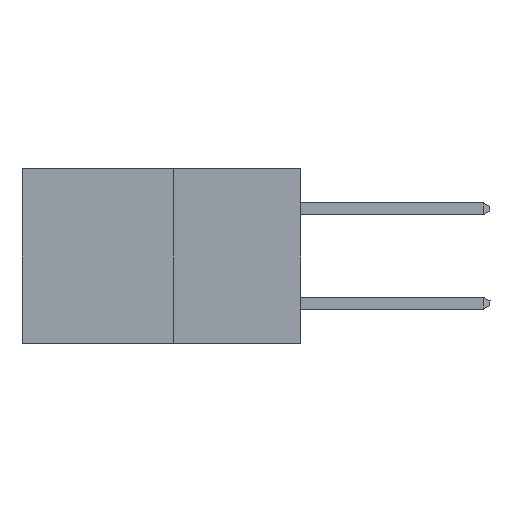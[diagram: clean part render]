
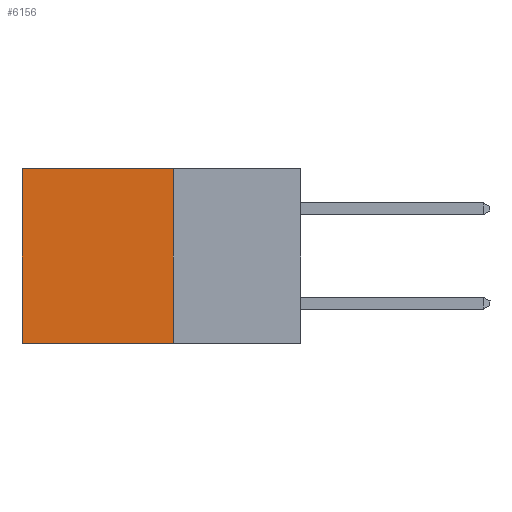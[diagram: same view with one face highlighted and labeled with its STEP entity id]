
A CAD part, left-side view. The second image highlights one B-rep face of the part: STEP entity #6156.
In plain terms, the highlighted planar face has unit normal (-1, 0, 0).
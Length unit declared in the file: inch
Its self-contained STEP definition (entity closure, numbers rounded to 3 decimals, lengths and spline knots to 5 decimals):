
#338 = DIRECTION ( 'NONE',  ( 0., 1., 0. ) ) ;
#773 = CARTESIAN_POINT ( 'NONE',  ( 0.277, 0.27, 0. ) ) ;
#1334 = CARTESIAN_POINT ( 'NONE',  ( 0.277, 0.59, -0.37 ) ) ;
#2252 = EDGE_CURVE ( 'NONE', #5925, #19746, #11909, .T. ) ;
#2557 = VECTOR ( 'NONE', #9888, 39.37008 ) ;
#2667 = VECTOR ( 'NONE', #3461, 39.37008 ) ;
#2923 = CARTESIAN_POINT ( 'NONE',  ( 0.277, 0.59, -0.37 ) ) ;
#3461 = DIRECTION ( 'NONE',  ( 0., 0., -1. ) ) ;
#3554 = CARTESIAN_POINT ( 'NONE',  ( 0.277, 0.27, -0.37 ) ) ;
#3560 = DIRECTION ( 'NONE',  ( 0., 1., 0. ) ) ;
#4590 = EDGE_CURVE ( 'NONE', #21267, #15709, #16274, .T. ) ;
#5071 = EDGE_CURVE ( 'NONE', #21267, #5925, #7165, .T. ) ;
#5925 = VERTEX_POINT ( 'NONE', #18379 ) ;
#6156 = ADVANCED_FACE ( 'NONE', ( #7928 ), #14981, .F. ) ;
#7165 = LINE ( 'NONE', #773, #20092 ) ;
#7708 = EDGE_LOOP ( 'NONE', ( #18186, #8403, #14616, #10202 ) ) ;
#7849 = LINE ( 'NONE', #3554, #19721 ) ;
#7928 = FACE_OUTER_BOUND ( 'NONE', #7708, .T. ) ;
#7953 = EDGE_CURVE ( 'NONE', #15709, #19746, #7849, .T. ) ;
#8391 = CARTESIAN_POINT ( 'NONE',  ( 0.277, 0.27, -0.37 ) ) ;
#8403 = ORIENTED_EDGE ( 'NONE', *, *, #7953, .F. ) ;
#9888 = DIRECTION ( 'NONE',  ( 0., 0., -1. ) ) ;
#10202 = ORIENTED_EDGE ( 'NONE', *, *, #5071, .T. ) ;
#10228 = CARTESIAN_POINT ( 'NONE',  ( 0.277, 0.27, -0.37 ) ) ;
#11780 = CARTESIAN_POINT ( 'NONE',  ( 0.277, 0.27, 0. ) ) ;
#11909 = LINE ( 'NONE', #2923, #2667 ) ;
#14616 = ORIENTED_EDGE ( 'NONE', *, *, #4590, .F. ) ;
#14844 = DIRECTION ( 'NONE',  ( 0., 0., -1. ) ) ;
#14861 = DIRECTION ( 'NONE',  ( 1., 0., 0. ) ) ;
#14950 = AXIS2_PLACEMENT_3D ( 'NONE', #15056, #14861, #14844 ) ;
#14981 = PLANE ( 'NONE',  #14950 ) ;
#15056 = CARTESIAN_POINT ( 'NONE',  ( 0.277, 0.27, -0.37 ) ) ;
#15709 = VERTEX_POINT ( 'NONE', #8391 ) ;
#16274 = LINE ( 'NONE', #10228, #2557 ) ;
#18186 = ORIENTED_EDGE ( 'NONE', *, *, #2252, .T. ) ;
#18379 = CARTESIAN_POINT ( 'NONE',  ( 0.277, 0.59, 0. ) ) ;
#19721 = VECTOR ( 'NONE', #3560, 39.37008 ) ;
#19746 = VERTEX_POINT ( 'NONE', #1334 ) ;
#20092 = VECTOR ( 'NONE', #338, 39.37008 ) ;
#21267 = VERTEX_POINT ( 'NONE', #11780 ) ;
